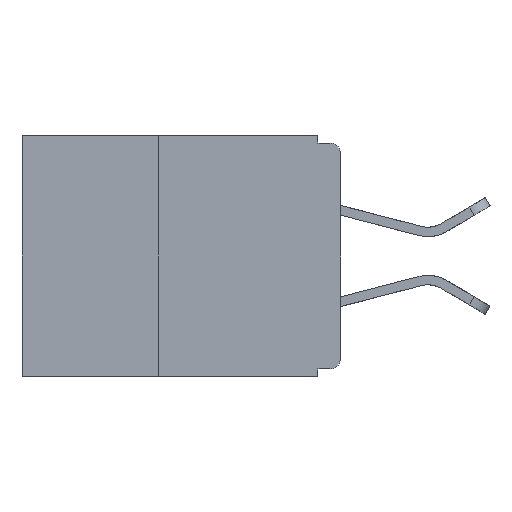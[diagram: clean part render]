
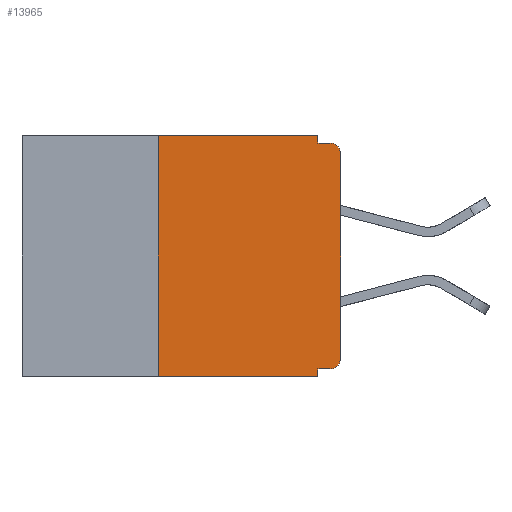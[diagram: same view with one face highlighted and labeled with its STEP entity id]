
A CAD part, left-side view. The second image highlights one B-rep face of the part: STEP entity #13965.
In plain terms, the highlighted planar face has unit normal (-1, 0, 0).
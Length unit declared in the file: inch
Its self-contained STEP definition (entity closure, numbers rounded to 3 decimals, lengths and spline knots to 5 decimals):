
#83 = DIRECTION ( 'NONE',  ( 0., 0., -1. ) ) ;
#233 = VECTOR ( 'NONE', #10878, 39.37008 ) ;
#333 = LINE ( 'NONE', #460, #25376 ) ;
#341 = AXIS2_PLACEMENT_3D ( 'NONE', #26694, #12308, #29082 ) ;
#460 = CARTESIAN_POINT ( 'NONE',  ( 0., 0.437, 0. ) ) ;
#1190 = CARTESIAN_POINT ( 'NONE',  ( 0., 0.015, -0.01 ) ) ;
#1440 = VERTEX_POINT ( 'NONE', #30198 ) ;
#1491 = LINE ( 'NONE', #2985, #31247 ) ;
#2080 = DIRECTION ( 'NONE',  ( 0., 0., -1. ) ) ;
#2140 = VECTOR ( 'NONE', #15339, 39.37008 ) ;
#2239 = VERTEX_POINT ( 'NONE', #6759 ) ;
#2329 = CARTESIAN_POINT ( 'NONE',  ( 0., 0., -0.01 ) ) ;
#2463 = EDGE_CURVE ( 'NONE', #28069, #7465, #14370, .T. ) ;
#2856 = EDGE_CURVE ( 'NONE', #27951, #17463, #6798, .T. ) ;
#2985 = CARTESIAN_POINT ( 'NONE',  ( 0., 0., 0. ) ) ;
#3570 = CARTESIAN_POINT ( 'NONE',  ( 0., 0.25, 0. ) ) ;
#3655 = AXIS2_PLACEMENT_3D ( 'NONE', #29080, #14734, #83 ) ;
#4097 = LINE ( 'NONE', #2329, #21889 ) ;
#5303 = EDGE_CURVE ( 'NONE', #7195, #11344, #7782, .T. ) ;
#5942 = DIRECTION ( 'NONE',  ( 0., 1., 0. ) ) ;
#6759 = CARTESIAN_POINT ( 'NONE',  ( 0., 0.015, -0.32 ) ) ;
#6785 = CARTESIAN_POINT ( 'NONE',  ( 0., 0., -0.305 ) ) ;
#6798 = LINE ( 'NONE', #12639, #233 ) ;
#6916 = CARTESIAN_POINT ( 'NONE',  ( 0., 0.437, 0. ) ) ;
#7195 = VERTEX_POINT ( 'NONE', #16485 ) ;
#7262 = DIRECTION ( 'NONE',  ( 0., -1., 0. ) ) ;
#7436 = EDGE_CURVE ( 'NONE', #17463, #7195, #333, .T. ) ;
#7465 = VERTEX_POINT ( 'NONE', #10347 ) ;
#7552 = AXIS2_PLACEMENT_3D ( 'NONE', #6916, #16667, #2080 ) ;
#7782 = LINE ( 'NONE', #18694, #19895 ) ;
#8328 = CARTESIAN_POINT ( 'NONE',  ( 0., 0.25, -0.33 ) ) ;
#8605 = ORIENTED_EDGE ( 'NONE', *, *, #2463, .F. ) ;
#8698 = CARTESIAN_POINT ( 'NONE',  ( 0., 0.031, -0.33 ) ) ;
#8831 = VECTOR ( 'NONE', #5942, 39.37008 ) ;
#8961 = CIRCLE ( 'NONE', #3655, 0.015 ) ;
#10347 = CARTESIAN_POINT ( 'NONE',  ( 0., 0.031, -0.33 ) ) ;
#10534 = EDGE_CURVE ( 'NONE', #11344, #19304, #4097, .T. ) ;
#10878 = DIRECTION ( 'NONE',  ( 0., 0., 1. ) ) ;
#11211 = CARTESIAN_POINT ( 'NONE',  ( 0., 0.031, -0.32 ) ) ;
#11274 = ORIENTED_EDGE ( 'NONE', *, *, #2856, .F. ) ;
#11344 = VERTEX_POINT ( 'NONE', #12654 ) ;
#11878 = EDGE_CURVE ( 'NONE', #1440, #19304, #8961, .T. ) ;
#12308 = DIRECTION ( 'NONE',  ( -1., 0., 0. ) ) ;
#12639 = CARTESIAN_POINT ( 'NONE',  ( 0., 0.25, -0.33 ) ) ;
#12654 = CARTESIAN_POINT ( 'NONE',  ( 0., 0.031, -0.01 ) ) ;
#12657 = VERTEX_POINT ( 'NONE', #6785 ) ;
#12773 = ORIENTED_EDGE ( 'NONE', *, *, #30695, .T. ) ;
#12792 = DIRECTION ( 'NONE',  ( 0., 0., 1. ) ) ;
#12896 = CARTESIAN_POINT ( 'NONE',  ( 0., 0.437, -0.33 ) ) ;
#13045 = FACE_OUTER_BOUND ( 'NONE', #28027, .T. ) ;
#13608 = VECTOR ( 'NONE', #27341, 39.37008 ) ;
#13965 = ADVANCED_FACE ( 'NONE', ( #13045 ), #30926, .F. ) ;
#14325 = ORIENTED_EDGE ( 'NONE', *, *, #5303, .F. ) ;
#14370 = LINE ( 'NONE', #8698, #13608 ) ;
#14734 = DIRECTION ( 'NONE',  ( -1., 0., 0. ) ) ;
#15339 = DIRECTION ( 'NONE',  ( 0., -1., 0. ) ) ;
#15454 = ORIENTED_EDGE ( 'NONE', *, *, #27062, .T. ) ;
#15603 = CARTESIAN_POINT ( 'NONE',  ( 0., 0., -0.32 ) ) ;
#16009 = LINE ( 'NONE', #15603, #8831 ) ;
#16033 = ORIENTED_EDGE ( 'NONE', *, *, #21674, .T. ) ;
#16485 = CARTESIAN_POINT ( 'NONE',  ( 0., 0.031, 0. ) ) ;
#16667 = DIRECTION ( 'NONE',  ( 1., 0., 0. ) ) ;
#17195 = CIRCLE ( 'NONE', #341, 0.015 ) ;
#17463 = VERTEX_POINT ( 'NONE', #3570 ) ;
#18490 = DIRECTION ( 'NONE',  ( 0., 0., -1. ) ) ;
#18694 = CARTESIAN_POINT ( 'NONE',  ( 0., 0.031, 0. ) ) ;
#19304 = VERTEX_POINT ( 'NONE', #1190 ) ;
#19895 = VECTOR ( 'NONE', #18490, 39.37008 ) ;
#19952 = DIRECTION ( 'NONE',  ( 0., -1., 0. ) ) ;
#21529 = LINE ( 'NONE', #12896, #2140 ) ;
#21674 = EDGE_CURVE ( 'NONE', #12657, #1440, #1491, .T. ) ;
#21889 = VECTOR ( 'NONE', #7262, 39.37008 ) ;
#22625 = ORIENTED_EDGE ( 'NONE', *, *, #11878, .T. ) ;
#24098 = ORIENTED_EDGE ( 'NONE', *, *, #10534, .F. ) ;
#24447 = ORIENTED_EDGE ( 'NONE', *, *, #28572, .F. ) ;
#25376 = VECTOR ( 'NONE', #19952, 39.37008 ) ;
#26694 = CARTESIAN_POINT ( 'NONE',  ( 0., 0.015, -0.305 ) ) ;
#27062 = EDGE_CURVE ( 'NONE', #2239, #12657, #17195, .T. ) ;
#27341 = DIRECTION ( 'NONE',  ( 0., 0., -1. ) ) ;
#27951 = VERTEX_POINT ( 'NONE', #8328 ) ;
#28027 = EDGE_LOOP ( 'NONE', ( #16033, #22625, #24098, #14325, #29637, #11274, #12773, #8605, #24447, #15454 ) ) ;
#28069 = VERTEX_POINT ( 'NONE', #11211 ) ;
#28572 = EDGE_CURVE ( 'NONE', #2239, #28069, #16009, .T. ) ;
#29080 = CARTESIAN_POINT ( 'NONE',  ( 0., 0.015, -0.025 ) ) ;
#29082 = DIRECTION ( 'NONE',  ( 0., 0., -1. ) ) ;
#29637 = ORIENTED_EDGE ( 'NONE', *, *, #7436, .F. ) ;
#30198 = CARTESIAN_POINT ( 'NONE',  ( 0., 0., -0.025 ) ) ;
#30695 = EDGE_CURVE ( 'NONE', #27951, #7465, #21529, .T. ) ;
#30926 = PLANE ( 'NONE',  #7552 ) ;
#31247 = VECTOR ( 'NONE', #12792, 39.37008 ) ;
